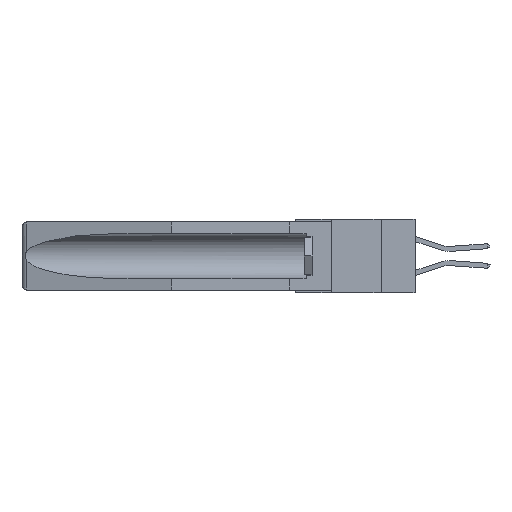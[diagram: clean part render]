
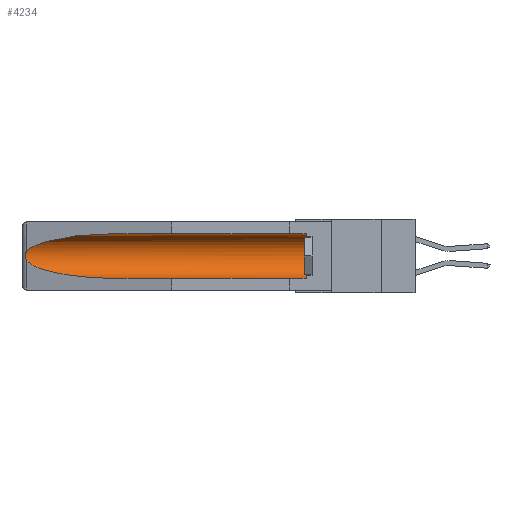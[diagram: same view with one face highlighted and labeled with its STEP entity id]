
A CAD part, left-side view. The second image highlights one B-rep face of the part: STEP entity #4234.
In plain terms, the highlighted cylindrical face has radius 2.857 mm (diameter 5.715 mm), a partial arc.
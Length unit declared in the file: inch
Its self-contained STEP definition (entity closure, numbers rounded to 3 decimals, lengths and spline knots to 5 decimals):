
#102 = LINE ( 'NONE', #17755, #8119 ) ;
#229 = CARTESIAN_POINT ( 'NONE',  ( 0.2673, 1.53269, -0.17917 ) ) ;
#361 = CARTESIAN_POINT ( 'NONE',  ( 0.2675, 1.53308, -0.17534 ) ) ;
#422 = AXIS2_PLACEMENT_3D ( 'NONE', #9404, #3815, #15049 ) ;
#562 = B_SPLINE_CURVE_WITH_KNOTS ( 'NONE', 3,
 ( #3211, #7454, #15893, #11775, #7327, #361, #229, #7390, #3270, #10159 ),
 .UNSPECIFIED., .F., .F.,
 ( 4, 2, 2, 2, 4 ),
 ( 0., 0.00029, 0.00058, 0.00087, 0.00117 ),
 .UNSPECIFIED. ) ;
#639 = DIRECTION ( 'NONE',  ( 0., 1., 0. ) ) ;
#1239 = EDGE_CURVE ( 'NONE', #9513, #3245, #10947, .T. ) ;
#2121 = FACE_OUTER_BOUND ( 'NONE', #17284, .T. ) ;
#2634 = VECTOR ( 'NONE', #18066, 39.37008 ) ;
#3143 = AXIS2_PLACEMENT_3D ( 'NONE', #5614, #14219, #15593 ) ;
#3211 = CARTESIAN_POINT ( 'NONE',  ( 0.26537, 1.52718, -0.14972 ) ) ;
#3245 = VERTEX_POINT ( 'NONE', #13729 ) ;
#3270 = CARTESIAN_POINT ( 'NONE',  ( 0.26597, 1.5296, -0.19026 ) ) ;
#3815 = DIRECTION ( 'NONE',  ( 0., 1., 0. ) ) ;
#4118 =( BOUNDED_CURVE ( )  B_SPLINE_CURVE ( 3, ( #5873, #17372, #7491, #13222 ),
 .UNSPECIFIED., .F., .F. ) 
 B_SPLINE_CURVE_WITH_KNOTS ( ( 4, 4 ),
 ( 4.71239, 6.08839 ),
 .UNSPECIFIED. ) 
 CURVE ( )  GEOMETRIC_REPRESENTATION_ITEM ( )  RATIONAL_B_SPLINE_CURVE ( ( 1., 0.848, 0.848, 1. ) ) 
 REPRESENTATION_ITEM ( '' )  );
#4146 = CYLINDRICAL_SURFACE ( 'NONE', #422, 0.1125 ) ;
#4234 = ADVANCED_FACE ( 'NONE', ( #2121 ), #4146, .F. ) ;
#4818 = VERTEX_POINT ( 'NONE', #15732 ) ;
#4982 = VERTEX_POINT ( 'NONE', #17246 ) ;
#5492 = ORIENTED_EDGE ( 'NONE', *, *, #10930, .F. ) ;
#5614 = CARTESIAN_POINT ( 'NONE',  ( 0.155, 0.126, -0.1715 ) ) ;
#5873 = CARTESIAN_POINT ( 'NONE',  ( 0.155, 1.07973, -0.059 ) ) ;
#7327 = CARTESIAN_POINT ( 'NONE',  ( 0.2675, 1.53308, -0.16763 ) ) ;
#7390 = CARTESIAN_POINT ( 'NONE',  ( 0.26655, 1.53094, -0.18657 ) ) ;
#7454 = CARTESIAN_POINT ( 'NONE',  ( 0.26597, 1.52961, -0.15275 ) ) ;
#7491 = CARTESIAN_POINT ( 'NONE',  ( 0.25451, 1.48313, -0.09465 ) ) ;
#7525 = ORIENTED_EDGE ( 'NONE', *, *, #14133, .T. ) ;
#8119 = VECTOR ( 'NONE', #639, 39.37008 ) ;
#8333 = VERTEX_POINT ( 'NONE', #10612 ) ;
#8490 = EDGE_CURVE ( 'NONE', #4818, #8333, #11851, .T. ) ;
#9092 = LINE ( 'NONE', #13805, #2634 ) ;
#9110 = CARTESIAN_POINT ( 'NONE',  ( 0.26537, 1.52718, -0.19328 ) ) ;
#9255 = EDGE_CURVE ( 'NONE', #14860, #4818, #562, .T. ) ;
#9404 = CARTESIAN_POINT ( 'NONE',  ( 0.155, -0.30754, -0.1715 ) ) ;
#9513 = VERTEX_POINT ( 'NONE', #10054 ) ;
#9975 = CARTESIAN_POINT ( 'NONE',  ( 0.155, 1.07973, -0.284 ) ) ;
#10054 = CARTESIAN_POINT ( 'NONE',  ( 0.155, 0.126, -0.284 ) ) ;
#10159 = CARTESIAN_POINT ( 'NONE',  ( 0.26537, 1.52718, -0.19328 ) ) ;
#10612 = CARTESIAN_POINT ( 'NONE',  ( 0.155, 1.07973, -0.284 ) ) ;
#10930 = EDGE_CURVE ( 'NONE', #9513, #8333, #102, .T. ) ;
#10947 = CIRCLE ( 'NONE', #3143, 0.1125 ) ;
#11280 = ORIENTED_EDGE ( 'NONE', *, *, #15550, .T. ) ;
#11370 = ORIENTED_EDGE ( 'NONE', *, *, #9255, .T. ) ;
#11775 = CARTESIAN_POINT ( 'NONE',  ( 0.2673, 1.5327, -0.16383 ) ) ;
#11851 =( BOUNDED_CURVE ( )  B_SPLINE_CURVE ( 3, ( #9110, #12113, #15638, #9975 ),
 .UNSPECIFIED., .F., .F. ) 
 B_SPLINE_CURVE_WITH_KNOTS ( ( 4, 4 ),
 ( 0.1948, 1.5708 ),
 .UNSPECIFIED. ) 
 CURVE ( )  GEOMETRIC_REPRESENTATION_ITEM ( )  RATIONAL_B_SPLINE_CURVE ( ( 1., 0.848, 0.848, 1. ) ) 
 REPRESENTATION_ITEM ( '' )  );
#12113 = CARTESIAN_POINT ( 'NONE',  ( 0.25451, 1.48313, -0.24835 ) ) ;
#12881 = ORIENTED_EDGE ( 'NONE', *, *, #1239, .T. ) ;
#13222 = CARTESIAN_POINT ( 'NONE',  ( 0.26537, 1.52718, -0.14972 ) ) ;
#13729 = CARTESIAN_POINT ( 'NONE',  ( 0.155, 0.126, -0.059 ) ) ;
#13805 = CARTESIAN_POINT ( 'NONE',  ( 0.155, -0.30754, -0.059 ) ) ;
#14133 = EDGE_CURVE ( 'NONE', #3245, #4982, #9092, .T. ) ;
#14219 = DIRECTION ( 'NONE',  ( 0., -1., 0. ) ) ;
#14860 = VERTEX_POINT ( 'NONE', #16659 ) ;
#15049 = DIRECTION ( 'NONE',  ( 0., 0., 1. ) ) ;
#15550 = EDGE_CURVE ( 'NONE', #4982, #14860, #4118, .T. ) ;
#15593 = DIRECTION ( 'NONE',  ( 0., 0., 1. ) ) ;
#15638 = CARTESIAN_POINT ( 'NONE',  ( 0.21114, 1.30732, -0.284 ) ) ;
#15732 = CARTESIAN_POINT ( 'NONE',  ( 0.26537, 1.52718, -0.19328 ) ) ;
#15893 = CARTESIAN_POINT ( 'NONE',  ( 0.26654, 1.53092, -0.15636 ) ) ;
#16659 = CARTESIAN_POINT ( 'NONE',  ( 0.26537, 1.52718, -0.14972 ) ) ;
#17246 = CARTESIAN_POINT ( 'NONE',  ( 0.155, 1.07973, -0.059 ) ) ;
#17284 = EDGE_LOOP ( 'NONE', ( #11280, #11370, #18323, #5492, #12881, #7525 ) ) ;
#17372 = CARTESIAN_POINT ( 'NONE',  ( 0.21114, 1.30732, -0.059 ) ) ;
#17755 = CARTESIAN_POINT ( 'NONE',  ( 0.155, -0.30754, -0.284 ) ) ;
#18066 = DIRECTION ( 'NONE',  ( 0., 1., 0. ) ) ;
#18323 = ORIENTED_EDGE ( 'NONE', *, *, #8490, .T. ) ;
